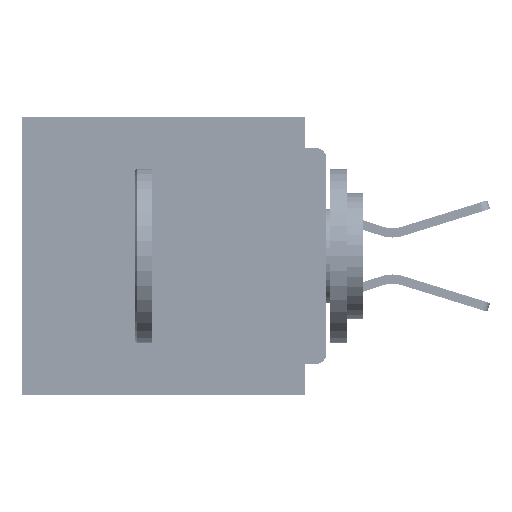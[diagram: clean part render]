
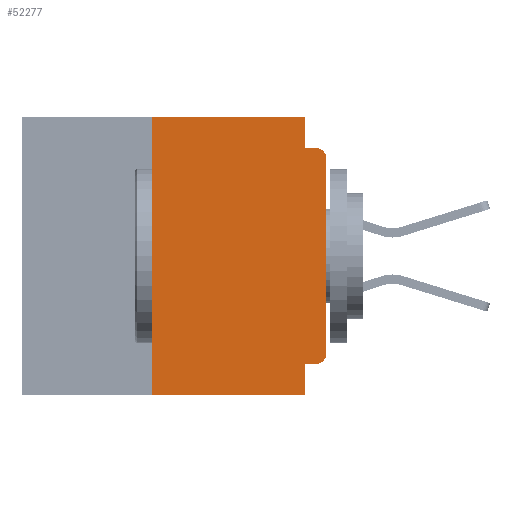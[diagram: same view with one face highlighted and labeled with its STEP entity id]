
A CAD part, left-side view. The second image highlights one B-rep face of the part: STEP entity #52277.
In plain terms, the highlighted planar face has unit normal (-1, 0, 0).
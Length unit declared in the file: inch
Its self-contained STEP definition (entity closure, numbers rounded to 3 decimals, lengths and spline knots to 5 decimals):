
#331 = VERTEX_POINT ( 'NONE', #59429 ) ;
#1133 = DIRECTION ( 'NONE',  ( 0., 0., -1. ) ) ;
#2988 = ORIENTED_EDGE ( 'NONE', *, *, #62360, .F. ) ;
#5649 = CARTESIAN_POINT ( 'NONE',  ( 0., 0., 0. ) ) ;
#6321 = EDGE_CURVE ( 'NONE', #11420, #331, #42809, .T. ) ;
#8701 = CARTESIAN_POINT ( 'NONE',  ( 0., 0., -0.045 ) ) ;
#9014 = CARTESIAN_POINT ( 'NONE',  ( 0., 0.031, -0.4 ) ) ;
#10343 = DIRECTION ( 'NONE',  ( 0., 0., -1. ) ) ;
#10945 = PLANE ( 'NONE',  #56378 ) ;
#11420 = VERTEX_POINT ( 'NONE', #22590 ) ;
#11633 = VECTOR ( 'NONE', #10343, 39.37008 ) ;
#12057 = ORIENTED_EDGE ( 'NONE', *, *, #58050, .T. ) ;
#12123 = AXIS2_PLACEMENT_3D ( 'NONE', #51146, #21641, #56114 ) ;
#12205 = CARTESIAN_POINT ( 'NONE',  ( 0., 0.015, -0.355 ) ) ;
#13157 = ORIENTED_EDGE ( 'NONE', *, *, #27834, .F. ) ;
#14921 = VECTOR ( 'NONE', #59913, 39.37008 ) ;
#15319 = CARTESIAN_POINT ( 'NONE',  ( 0., 0.031, 0. ) ) ;
#15935 = CARTESIAN_POINT ( 'NONE',  ( 0., 0.437, 0. ) ) ;
#16456 = LINE ( 'NONE', #35474, #14921 ) ;
#17046 = ORIENTED_EDGE ( 'NONE', *, *, #61096, .T. ) ;
#17103 = FACE_OUTER_BOUND ( 'NONE', #33993, .T. ) ;
#17460 = CARTESIAN_POINT ( 'NONE',  ( 0., 0.015, -0.06 ) ) ;
#19132 = CARTESIAN_POINT ( 'NONE',  ( 0., 0.25, 0. ) ) ;
#19286 = ORIENTED_EDGE ( 'NONE', *, *, #57626, .F. ) ;
#20867 = CARTESIAN_POINT ( 'NONE',  ( 0., 0.031, -0.4 ) ) ;
#21641 = DIRECTION ( 'NONE',  ( -1., 0., 0. ) ) ;
#22429 = DIRECTION ( 'NONE',  ( 0., 0., -1. ) ) ;
#22590 = CARTESIAN_POINT ( 'NONE',  ( 0., 0., -0.34 ) ) ;
#22707 = EDGE_CURVE ( 'NONE', #331, #46421, #62544, .T. ) ;
#23305 = LINE ( 'NONE', #15319, #11633 ) ;
#24284 = CIRCLE ( 'NONE', #12123, 0.015 ) ;
#24355 = EDGE_CURVE ( 'NONE', #35389, #28012, #27782, .T. ) ;
#25335 = CARTESIAN_POINT ( 'NONE',  ( 0., 0.031, 0. ) ) ;
#25909 = CARTESIAN_POINT ( 'NONE',  ( 0., 0.031, -0.045 ) ) ;
#26222 = VECTOR ( 'NONE', #40339, 39.37008 ) ;
#27782 = LINE ( 'NONE', #35430, #26222 ) ;
#27834 = EDGE_CURVE ( 'NONE', #28012, #61062, #48143, .T. ) ;
#28012 = VERTEX_POINT ( 'NONE', #19132 ) ;
#28018 = CARTESIAN_POINT ( 'NONE',  ( 0., 0.437, 0. ) ) ;
#29597 = VERTEX_POINT ( 'NONE', #12205 ) ;
#30869 = DIRECTION ( 'NONE',  ( 1., 0., 0. ) ) ;
#33001 = CARTESIAN_POINT ( 'NONE',  ( 0., 0.031, -0.355 ) ) ;
#33993 = EDGE_LOOP ( 'NONE', ( #51782, #54124, #2988, #44957, #13157, #55676, #17046, #61868, #19286, #12057 ) ) ;
#35314 = DIRECTION ( 'NONE',  ( 0., 0., 1. ) ) ;
#35389 = VERTEX_POINT ( 'NONE', #43543 ) ;
#35430 = CARTESIAN_POINT ( 'NONE',  ( 0., 0.25, -0.4 ) ) ;
#35474 = CARTESIAN_POINT ( 'NONE',  ( 0., 0.437, -0.4 ) ) ;
#37400 = LINE ( 'NONE', #20867, #48930 ) ;
#37893 = VECTOR ( 'NONE', #53158, 39.37008 ) ;
#38258 = CARTESIAN_POINT ( 'NONE',  ( 0., 0.015, -0.045 ) ) ;
#39427 = EDGE_CURVE ( 'NONE', #61062, #48128, #23305, .T. ) ;
#40339 = DIRECTION ( 'NONE',  ( 0., 0., 1. ) ) ;
#40492 = LINE ( 'NONE', #62509, #50522 ) ;
#42809 = LINE ( 'NONE', #5649, #54396 ) ;
#43045 = DIRECTION ( 'NONE',  ( 0., 1., 0. ) ) ;
#43543 = CARTESIAN_POINT ( 'NONE',  ( 0., 0.25, -0.4 ) ) ;
#44957 = ORIENTED_EDGE ( 'NONE', *, *, #39427, .F. ) ;
#46421 = VERTEX_POINT ( 'NONE', #38258 ) ;
#48128 = VERTEX_POINT ( 'NONE', #25909 ) ;
#48143 = LINE ( 'NONE', #28018, #61170 ) ;
#48930 = VECTOR ( 'NONE', #55346, 39.37008 ) ;
#50227 = AXIS2_PLACEMENT_3D ( 'NONE', #17460, #51947, #22429 ) ;
#50522 = VECTOR ( 'NONE', #43045, 39.37008 ) ;
#50976 = LINE ( 'NONE', #8701, #37893 ) ;
#51146 = CARTESIAN_POINT ( 'NONE',  ( 0., 0.015, -0.34 ) ) ;
#51782 = ORIENTED_EDGE ( 'NONE', *, *, #6321, .T. ) ;
#51947 = DIRECTION ( 'NONE',  ( -1., 0., 0. ) ) ;
#52277 = ADVANCED_FACE ( 'NONE', ( #17103 ), #10945, .F. ) ;
#53158 = DIRECTION ( 'NONE',  ( 0., -1., 0. ) ) ;
#54124 = ORIENTED_EDGE ( 'NONE', *, *, #22707, .T. ) ;
#54396 = VECTOR ( 'NONE', #35314, 39.37008 ) ;
#55346 = DIRECTION ( 'NONE',  ( 0., 0., -1. ) ) ;
#55676 = ORIENTED_EDGE ( 'NONE', *, *, #24355, .F. ) ;
#56114 = DIRECTION ( 'NONE',  ( 0., 0., -1. ) ) ;
#56378 = AXIS2_PLACEMENT_3D ( 'NONE', #15935, #30869, #1133 ) ;
#57081 = VERTEX_POINT ( 'NONE', #33001 ) ;
#57626 = EDGE_CURVE ( 'NONE', #29597, #57081, #40492, .T. ) ;
#58050 = EDGE_CURVE ( 'NONE', #29597, #11420, #24284, .T. ) ;
#59429 = CARTESIAN_POINT ( 'NONE',  ( 0., 0., -0.06 ) ) ;
#59913 = DIRECTION ( 'NONE',  ( 0., -1., 0. ) ) ;
#60519 = EDGE_CURVE ( 'NONE', #57081, #61964, #37400, .T. ) ;
#61062 = VERTEX_POINT ( 'NONE', #25335 ) ;
#61096 = EDGE_CURVE ( 'NONE', #35389, #61964, #16456, .T. ) ;
#61170 = VECTOR ( 'NONE', #62342, 39.37008 ) ;
#61868 = ORIENTED_EDGE ( 'NONE', *, *, #60519, .F. ) ;
#61964 = VERTEX_POINT ( 'NONE', #9014 ) ;
#62342 = DIRECTION ( 'NONE',  ( 0., -1., 0. ) ) ;
#62360 = EDGE_CURVE ( 'NONE', #48128, #46421, #50976, .T. ) ;
#62509 = CARTESIAN_POINT ( 'NONE',  ( 0., 0., -0.355 ) ) ;
#62544 = CIRCLE ( 'NONE', #50227, 0.015 ) ;
